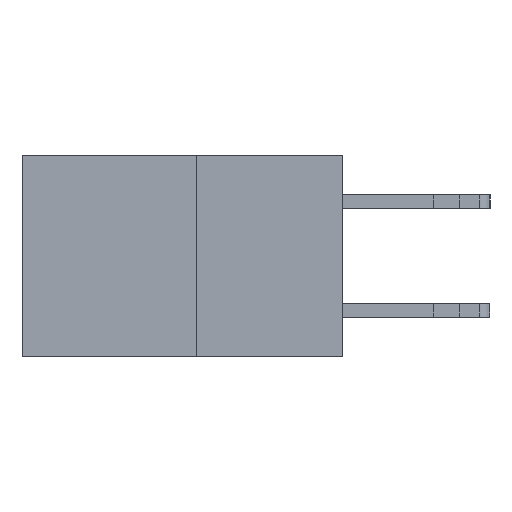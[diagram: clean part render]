
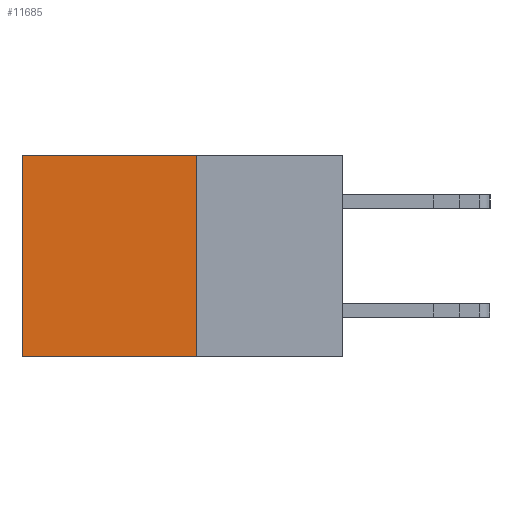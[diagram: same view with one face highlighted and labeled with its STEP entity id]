
A CAD part, left-side view. The second image highlights one B-rep face of the part: STEP entity #11685.
In plain terms, the highlighted planar face has unit normal (-1, 0, 0).
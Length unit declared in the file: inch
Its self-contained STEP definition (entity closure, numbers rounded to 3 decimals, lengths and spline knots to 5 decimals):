
#183 = LINE ( 'NONE', #16231, #7407 ) ;
#258 = VERTEX_POINT ( 'NONE', #11679 ) ;
#728 = DIRECTION ( 'NONE',  ( 1., 0., 0. ) ) ;
#1031 = EDGE_CURVE ( 'NONE', #2852, #13048, #12983, .T. ) ;
#1782 = CARTESIAN_POINT ( 'NONE',  ( 0.277, 0.27, -0.37 ) ) ;
#2852 = VERTEX_POINT ( 'NONE', #13244 ) ;
#3167 = DIRECTION ( 'NONE',  ( 0., 1., 0. ) ) ;
#3322 = AXIS2_PLACEMENT_3D ( 'NONE', #12721, #728, #10200 ) ;
#4201 = FACE_OUTER_BOUND ( 'NONE', #5616, .T. ) ;
#4429 = CARTESIAN_POINT ( 'NONE',  ( 0.277, 0.59, -0.37 ) ) ;
#5616 = EDGE_LOOP ( 'NONE', ( #9072, #15411, #15571, #16856 ) ) ;
#7407 = VECTOR ( 'NONE', #9754, 39.37008 ) ;
#7917 = EDGE_CURVE ( 'NONE', #258, #16287, #16715, .T. ) ;
#7920 = CARTESIAN_POINT ( 'NONE',  ( 0.277, 0.59, 0. ) ) ;
#8057 = CARTESIAN_POINT ( 'NONE',  ( 0.277, 0.27, 0. ) ) ;
#8060 = CARTESIAN_POINT ( 'NONE',  ( 0.277, 0.59, -0.37 ) ) ;
#8304 = DIRECTION ( 'NONE',  ( 0., 1., 0. ) ) ;
#8809 = PLANE ( 'NONE',  #3322 ) ;
#9072 = ORIENTED_EDGE ( 'NONE', *, *, #12659, .T. ) ;
#9754 = DIRECTION ( 'NONE',  ( 0., 0., -1. ) ) ;
#10200 = DIRECTION ( 'NONE',  ( 0., 0., -1. ) ) ;
#10793 = EDGE_CURVE ( 'NONE', #2852, #258, #183, .T. ) ;
#11679 = CARTESIAN_POINT ( 'NONE',  ( 0.277, 0.27, -0.37 ) ) ;
#11685 = ADVANCED_FACE ( 'NONE', ( #4201 ), #8809, .F. ) ;
#12403 = DIRECTION ( 'NONE',  ( 0., 0., -1. ) ) ;
#12659 = EDGE_CURVE ( 'NONE', #13048, #16287, #16744, .T. ) ;
#12721 = CARTESIAN_POINT ( 'NONE',  ( 0.277, 0.27, -0.37 ) ) ;
#12983 = LINE ( 'NONE', #8057, #16453 ) ;
#13048 = VERTEX_POINT ( 'NONE', #7920 ) ;
#13244 = CARTESIAN_POINT ( 'NONE',  ( 0.277, 0.27, 0. ) ) ;
#13298 = VECTOR ( 'NONE', #12403, 39.37008 ) ;
#15411 = ORIENTED_EDGE ( 'NONE', *, *, #7917, .F. ) ;
#15571 = ORIENTED_EDGE ( 'NONE', *, *, #10793, .F. ) ;
#16231 = CARTESIAN_POINT ( 'NONE',  ( 0.277, 0.27, -0.37 ) ) ;
#16287 = VERTEX_POINT ( 'NONE', #8060 ) ;
#16327 = VECTOR ( 'NONE', #3167, 39.37008 ) ;
#16453 = VECTOR ( 'NONE', #8304, 39.37008 ) ;
#16715 = LINE ( 'NONE', #1782, #16327 ) ;
#16744 = LINE ( 'NONE', #4429, #13298 ) ;
#16856 = ORIENTED_EDGE ( 'NONE', *, *, #1031, .T. ) ;
